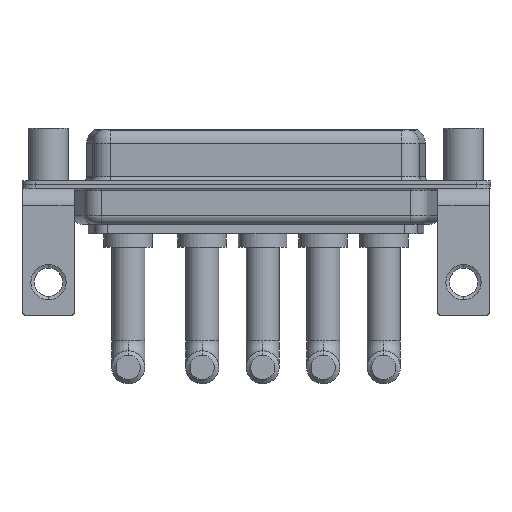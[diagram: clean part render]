
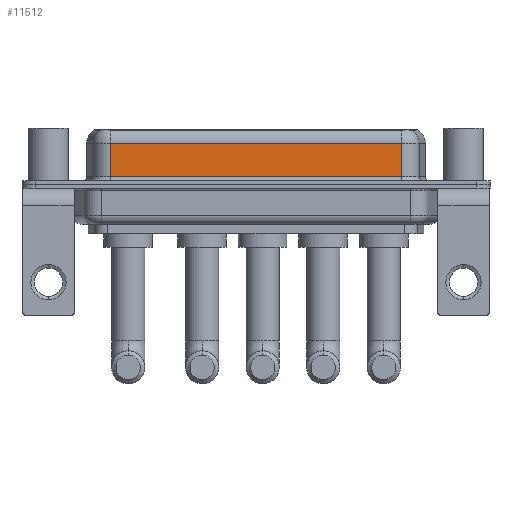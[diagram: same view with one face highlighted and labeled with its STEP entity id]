
A CAD part, front view. The second image highlights one B-rep face of the part: STEP entity #11512.
In plain terms, the highlighted planar face has unit normal (0, -1, 0).
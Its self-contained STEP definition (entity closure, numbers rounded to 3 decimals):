
#743 = DIRECTION ( 'NONE',  ( 0., 0., -1. ) ) ;
#1108 = LINE ( 'NONE', #11755, #6274 ) ;
#1621 = CARTESIAN_POINT ( 'NONE',  ( 40.037, -3.95, 4.65 ) ) ;
#1954 = ORIENTED_EDGE ( 'NONE', *, *, #10762, .T. ) ;
#2077 = CARTESIAN_POINT ( 'NONE',  ( 7.013, -3.95, 4.65 ) ) ;
#2207 = EDGE_CURVE ( 'NONE', #3523, #3288, #11382, .T. ) ;
#2660 = VERTEX_POINT ( 'NONE', #10986 ) ;
#2943 = VERTEX_POINT ( 'NONE', #2077 ) ;
#3288 = VERTEX_POINT ( 'NONE', #3697 ) ;
#3523 = VERTEX_POINT ( 'NONE', #8876 ) ;
#3697 = CARTESIAN_POINT ( 'NONE',  ( 40.037, -3.95, 0.9 ) ) ;
#4421 = DIRECTION ( 'NONE',  ( 0., 1., 0. ) ) ;
#4483 = AXIS2_PLACEMENT_3D ( 'NONE', #7971, #4421, #12912 ) ;
#5162 = DIRECTION ( 'NONE',  ( -1., 0., 0. ) ) ;
#6274 = VECTOR ( 'NONE', #9520, 1000. ) ;
#6727 = PLANE ( 'NONE',  #4483 ) ;
#6912 = ORIENTED_EDGE ( 'NONE', *, *, #9011, .T. ) ;
#7308 = EDGE_LOOP ( 'NONE', ( #14812, #6912, #10226, #1954 ) ) ;
#7463 = LINE ( 'NONE', #9788, #13607 ) ;
#7477 = LINE ( 'NONE', #1621, #8105 ) ;
#7739 = EDGE_CURVE ( 'NONE', #2943, #2660, #1108, .T. ) ;
#7971 = CARTESIAN_POINT ( 'NONE',  ( 40.037, -3.95, 6.4 ) ) ;
#8105 = VECTOR ( 'NONE', #5162, 1000. ) ;
#8876 = CARTESIAN_POINT ( 'NONE',  ( 40.037, -3.95, 4.65 ) ) ;
#9011 = EDGE_CURVE ( 'NONE', #3523, #2943, #7477, .T. ) ;
#9281 = FACE_OUTER_BOUND ( 'NONE', #7308, .T. ) ;
#9520 = DIRECTION ( 'NONE',  ( 0., 0., -1. ) ) ;
#9788 = CARTESIAN_POINT ( 'NONE',  ( 40.037, -3.95, 0.9 ) ) ;
#10226 = ORIENTED_EDGE ( 'NONE', *, *, #7739, .T. ) ;
#10762 = EDGE_CURVE ( 'NONE', #2660, #3288, #7463, .T. ) ;
#10986 = CARTESIAN_POINT ( 'NONE',  ( 7.013, -3.95, 0.9 ) ) ;
#11014 = VECTOR ( 'NONE', #743, 1000. ) ;
#11382 = LINE ( 'NONE', #14709, #11014 ) ;
#11512 = ADVANCED_FACE ( 'NONE', ( #9281 ), #6727, .F. ) ;
#11755 = CARTESIAN_POINT ( 'NONE',  ( 7.013, -3.95, 6.4 ) ) ;
#12912 = DIRECTION ( 'NONE',  ( 0., 0., 1. ) ) ;
#13607 = VECTOR ( 'NONE', #14261, 1000. ) ;
#14261 = DIRECTION ( 'NONE',  ( 1., 0., 0. ) ) ;
#14709 = CARTESIAN_POINT ( 'NONE',  ( 40.037, -3.95, 6.4 ) ) ;
#14812 = ORIENTED_EDGE ( 'NONE', *, *, #2207, .F. ) ;
